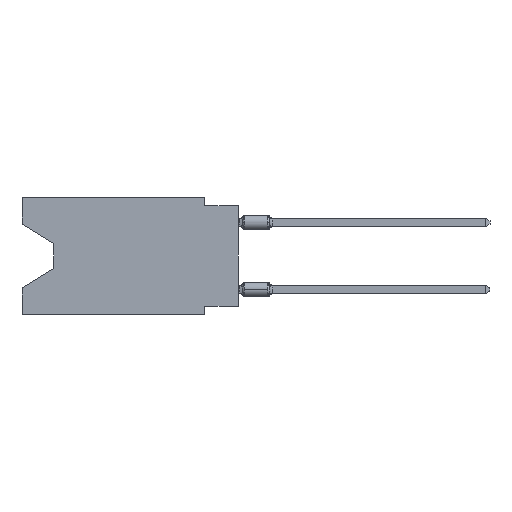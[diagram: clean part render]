
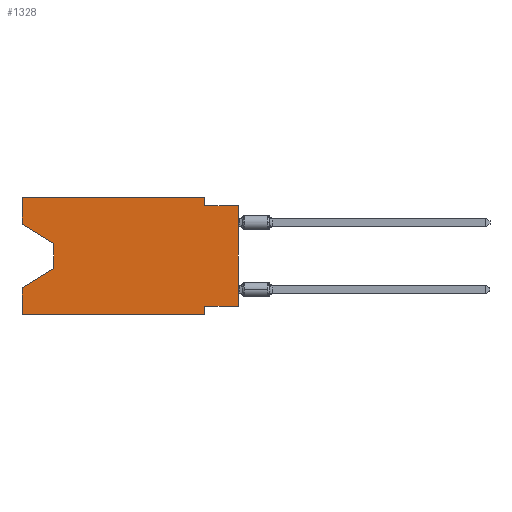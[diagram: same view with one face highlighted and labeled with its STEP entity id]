
A CAD part, left-side view. The second image highlights one B-rep face of the part: STEP entity #1328.
In plain terms, the highlighted planar face has unit normal (-1, 0, 0).
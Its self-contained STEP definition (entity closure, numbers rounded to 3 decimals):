
#45 = VERTEX_POINT ( 'NONE', #338 ) ;
#100 = DIRECTION ( 'NONE',  ( 0., -1., 0. ) ) ;
#248 = LINE ( 'NONE', #5422, #2537 ) ;
#338 = CARTESIAN_POINT ( 'NONE',  ( 0., 2.54, -8.255 ) ) ;
#410 = VECTOR ( 'NONE', #100, 1000. ) ;
#673 = CARTESIAN_POINT ( 'NONE',  ( 0., 16.383, -2.038 ) ) ;
#684 = CARTESIAN_POINT ( 'NONE',  ( 0., 0., -8.255 ) ) ;
#815 = EDGE_LOOP ( 'NONE', ( #3507, #5501, #7798, #4720, #7987, #5977, #10420, #4431, #6189, #8218, #967, #5972 ) ) ;
#967 = ORIENTED_EDGE ( 'NONE', *, *, #16442, .F. ) ;
#1163 = VERTEX_POINT ( 'NONE', #7871 ) ;
#1328 = ADVANCED_FACE ( 'NONE', ( #3514 ), #13554, .F. ) ;
#1476 = DIRECTION ( 'NONE',  ( 0., 0., 1. ) ) ;
#1825 = CARTESIAN_POINT ( 'NONE',  ( 0., 16.383, 0. ) ) ;
#2212 = EDGE_CURVE ( 'NONE', #13961, #45, #12573, .T. ) ;
#2537 = VECTOR ( 'NONE', #12993, 1000. ) ;
#2648 = LINE ( 'NONE', #7817, #410 ) ;
#2717 = CARTESIAN_POINT ( 'NONE',  ( 0., 13.97, -5.385 ) ) ;
#2882 = VERTEX_POINT ( 'NONE', #5814 ) ;
#2965 = LINE ( 'NONE', #673, #8342 ) ;
#3246 = VECTOR ( 'NONE', #10003, 1000. ) ;
#3507 = ORIENTED_EDGE ( 'NONE', *, *, #10527, .T. ) ;
#3514 = FACE_OUTER_BOUND ( 'NONE', #815, .T. ) ;
#3583 = CARTESIAN_POINT ( 'NONE',  ( 0., 13.97, -3.505 ) ) ;
#3792 = LINE ( 'NONE', #7683, #4371 ) ;
#3897 = CARTESIAN_POINT ( 'NONE',  ( 0., 2.54, -8.89 ) ) ;
#4224 = VECTOR ( 'NONE', #4999, 1000. ) ;
#4371 = VECTOR ( 'NONE', #12882, 1000. ) ;
#4431 = ORIENTED_EDGE ( 'NONE', *, *, #8381, .T. ) ;
#4694 = DIRECTION ( 'NONE',  ( 0., 0., -1. ) ) ;
#4720 = ORIENTED_EDGE ( 'NONE', *, *, #10395, .F. ) ;
#4831 = CARTESIAN_POINT ( 'NONE',  ( 0., 16.383, -2.038 ) ) ;
#4999 = DIRECTION ( 'NONE',  ( 0., -1., 0. ) ) ;
#5315 = LINE ( 'NONE', #9217, #13439 ) ;
#5422 = CARTESIAN_POINT ( 'NONE',  ( 0., 16.383, 0. ) ) ;
#5501 = ORIENTED_EDGE ( 'NONE', *, *, #8585, .T. ) ;
#5814 = CARTESIAN_POINT ( 'NONE',  ( 0., 0., -0.635 ) ) ;
#5972 = ORIENTED_EDGE ( 'NONE', *, *, #15399, .F. ) ;
#5977 = ORIENTED_EDGE ( 'NONE', *, *, #12497, .F. ) ;
#6024 = DIRECTION ( 'NONE',  ( 0., 1., 0. ) ) ;
#6189 = ORIENTED_EDGE ( 'NONE', *, *, #12530, .F. ) ;
#6467 = CARTESIAN_POINT ( 'NONE',  ( 0., 2.54, -0.635 ) ) ;
#6513 = VERTEX_POINT ( 'NONE', #6467 ) ;
#6700 = DIRECTION ( 'NONE',  ( 0., 0., 1. ) ) ;
#6714 = CARTESIAN_POINT ( 'NONE',  ( 0., 13.97, -3.505 ) ) ;
#6792 = EDGE_CURVE ( 'NONE', #11567, #10671, #16308, .T. ) ;
#6892 = VECTOR ( 'NONE', #1476, 1000. ) ;
#7683 = CARTESIAN_POINT ( 'NONE',  ( 0., 16.383, 0. ) ) ;
#7798 = ORIENTED_EDGE ( 'NONE', *, *, #6792, .T. ) ;
#7817 = CARTESIAN_POINT ( 'NONE',  ( 0., 16.383, -8.89 ) ) ;
#7871 = CARTESIAN_POINT ( 'NONE',  ( 0., 2.54, 0. ) ) ;
#7987 = ORIENTED_EDGE ( 'NONE', *, *, #8811, .T. ) ;
#8218 = ORIENTED_EDGE ( 'NONE', *, *, #14186, .F. ) ;
#8342 = VECTOR ( 'NONE', #9502, 1000. ) ;
#8381 = EDGE_CURVE ( 'NONE', #13961, #2882, #11674, .T. ) ;
#8585 = EDGE_CURVE ( 'NONE', #15030, #11567, #12433, .T. ) ;
#8811 = EDGE_CURVE ( 'NONE', #10698, #13271, #2648, .T. ) ;
#8855 = CARTESIAN_POINT ( 'NONE',  ( 0., 2.54, -8.89 ) ) ;
#9151 = DIRECTION ( 'NONE',  ( 0., 0., -1. ) ) ;
#9217 = CARTESIAN_POINT ( 'NONE',  ( 0., 2.54, 0. ) ) ;
#9502 = DIRECTION ( 'NONE',  ( 0., -0.855, -0.519 ) ) ;
#10003 = DIRECTION ( 'NONE',  ( 0., 0.855, -0.519 ) ) ;
#10269 = CARTESIAN_POINT ( 'NONE',  ( 0., 0., -8.255 ) ) ;
#10395 = EDGE_CURVE ( 'NONE', #10698, #10671, #12914, .T. ) ;
#10420 = ORIENTED_EDGE ( 'NONE', *, *, #2212, .F. ) ;
#10527 = EDGE_CURVE ( 'NONE', #11864, #15030, #2965, .T. ) ;
#10671 = VERTEX_POINT ( 'NONE', #16632 ) ;
#10698 = VERTEX_POINT ( 'NONE', #12646 ) ;
#11015 = AXIS2_PLACEMENT_3D ( 'NONE', #1825, #12531, #16107 ) ;
#11117 = CARTESIAN_POINT ( 'NONE',  ( 0., 13.97, -5.385 ) ) ;
#11567 = VERTEX_POINT ( 'NONE', #2717 ) ;
#11674 = LINE ( 'NONE', #13199, #6892 ) ;
#11785 = VECTOR ( 'NONE', #4694, 1000. ) ;
#11829 = VECTOR ( 'NONE', #9151, 1000. ) ;
#11864 = VERTEX_POINT ( 'NONE', #4831 ) ;
#11943 = DIRECTION ( 'NONE',  ( 0., 0., -1. ) ) ;
#12099 = VECTOR ( 'NONE', #6024, 1000. ) ;
#12433 = LINE ( 'NONE', #3583, #11785 ) ;
#12497 = EDGE_CURVE ( 'NONE', #45, #13271, #16558, .T. ) ;
#12530 = EDGE_CURVE ( 'NONE', #6513, #2882, #16638, .T. ) ;
#12531 = DIRECTION ( 'NONE',  ( 1., 0., 0. ) ) ;
#12573 = LINE ( 'NONE', #10269, #12099 ) ;
#12646 = CARTESIAN_POINT ( 'NONE',  ( 0., 16.383, -8.89 ) ) ;
#12713 = CARTESIAN_POINT ( 'NONE',  ( 0., 16.383, 0. ) ) ;
#12882 = DIRECTION ( 'NONE',  ( 0., -1., 0. ) ) ;
#12914 = LINE ( 'NONE', #15717, #15420 ) ;
#12993 = DIRECTION ( 'NONE',  ( 0., 0., 1. ) ) ;
#13199 = CARTESIAN_POINT ( 'NONE',  ( 0., 0., 0. ) ) ;
#13271 = VERTEX_POINT ( 'NONE', #8855 ) ;
#13439 = VECTOR ( 'NONE', #11943, 1000. ) ;
#13554 = PLANE ( 'NONE',  #11015 ) ;
#13961 = VERTEX_POINT ( 'NONE', #684 ) ;
#14186 = EDGE_CURVE ( 'NONE', #1163, #6513, #5315, .T. ) ;
#15030 = VERTEX_POINT ( 'NONE', #6714 ) ;
#15399 = EDGE_CURVE ( 'NONE', #11864, #16446, #248, .T. ) ;
#15420 = VECTOR ( 'NONE', #6700, 1000. ) ;
#15717 = CARTESIAN_POINT ( 'NONE',  ( 0., 16.383, 0. ) ) ;
#16107 = DIRECTION ( 'NONE',  ( 0., 0., -1. ) ) ;
#16308 = LINE ( 'NONE', #11117, #3246 ) ;
#16442 = EDGE_CURVE ( 'NONE', #16446, #1163, #3792, .T. ) ;
#16446 = VERTEX_POINT ( 'NONE', #12713 ) ;
#16558 = LINE ( 'NONE', #3897, #11829 ) ;
#16632 = CARTESIAN_POINT ( 'NONE',  ( 0., 16.383, -6.852 ) ) ;
#16638 = LINE ( 'NONE', #16727, #4224 ) ;
#16727 = CARTESIAN_POINT ( 'NONE',  ( 0., 0., -0.635 ) ) ;
